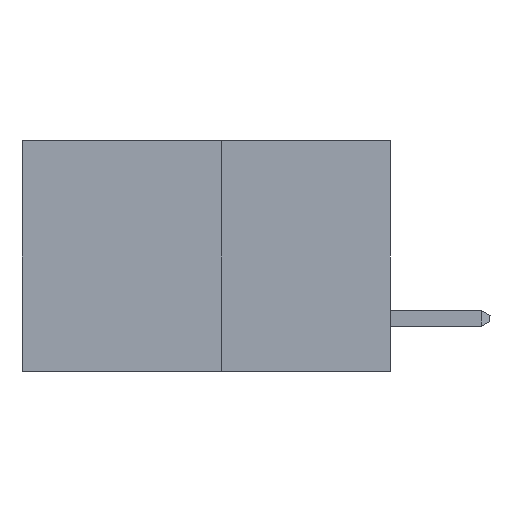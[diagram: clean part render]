
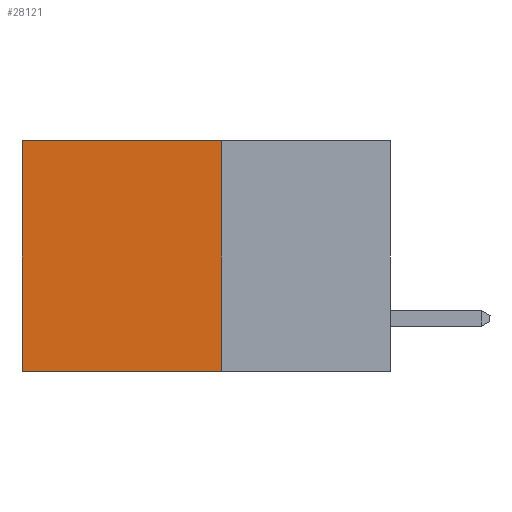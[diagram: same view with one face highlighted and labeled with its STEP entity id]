
A CAD part, left-side view. The second image highlights one B-rep face of the part: STEP entity #28121.
In plain terms, the highlighted planar face has unit normal (-1, 0, 0).
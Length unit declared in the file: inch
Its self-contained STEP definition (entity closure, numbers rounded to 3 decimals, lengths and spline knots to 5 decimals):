
#1997 = LINE ( 'NONE', #16569, #19466 ) ;
#2422 = DIRECTION ( 'NONE',  ( 0., 0., -1. ) ) ;
#3485 = CARTESIAN_POINT ( 'NONE',  ( 0.277, 0.59, 0. ) ) ;
#4413 = VERTEX_POINT ( 'NONE', #3485 ) ;
#4706 = CARTESIAN_POINT ( 'NONE',  ( 0.277, 0.27, -0.37 ) ) ;
#4904 = ORIENTED_EDGE ( 'NONE', *, *, #22801, .F. ) ;
#6611 = VERTEX_POINT ( 'NONE', #9168 ) ;
#7695 = CARTESIAN_POINT ( 'NONE',  ( 0.277, 0.27, -0.37 ) ) ;
#7754 = VERTEX_POINT ( 'NONE', #12438 ) ;
#8692 = EDGE_LOOP ( 'NONE', ( #22581, #11255, #4904, #27289 ) ) ;
#9168 = CARTESIAN_POINT ( 'NONE',  ( 0.277, 0.59, -0.37 ) ) ;
#9518 = CARTESIAN_POINT ( 'NONE',  ( 0.277, 0.59, -0.37 ) ) ;
#10011 = DIRECTION ( 'NONE',  ( 0., 1., 0. ) ) ;
#10153 = LINE ( 'NONE', #9518, #21510 ) ;
#11255 = ORIENTED_EDGE ( 'NONE', *, *, #15597, .F. ) ;
#12438 = CARTESIAN_POINT ( 'NONE',  ( 0.277, 0.27, -0.37 ) ) ;
#13337 = LINE ( 'NONE', #7695, #24687 ) ;
#14248 = DIRECTION ( 'NONE',  ( 0., 0., -1. ) ) ;
#14256 = CARTESIAN_POINT ( 'NONE',  ( 0.277, 0.27, 0. ) ) ;
#15376 = AXIS2_PLACEMENT_3D ( 'NONE', #18698, #27862, #14248 ) ;
#15597 = EDGE_CURVE ( 'NONE', #7754, #6611, #13337, .T. ) ;
#16569 = CARTESIAN_POINT ( 'NONE',  ( 0.277, 0.27, 0. ) ) ;
#17642 = VERTEX_POINT ( 'NONE', #14256 ) ;
#18698 = CARTESIAN_POINT ( 'NONE',  ( 0.277, 0.27, -0.37 ) ) ;
#18823 = DIRECTION ( 'NONE',  ( 0., 1., 0. ) ) ;
#19466 = VECTOR ( 'NONE', #18823, 39.37008 ) ;
#20769 = LINE ( 'NONE', #4706, #26132 ) ;
#20772 = EDGE_CURVE ( 'NONE', #17642, #4413, #1997, .T. ) ;
#21510 = VECTOR ( 'NONE', #25422, 39.37008 ) ;
#21965 = EDGE_CURVE ( 'NONE', #4413, #6611, #10153, .T. ) ;
#22581 = ORIENTED_EDGE ( 'NONE', *, *, #21965, .T. ) ;
#22801 = EDGE_CURVE ( 'NONE', #17642, #7754, #20769, .T. ) ;
#24246 = FACE_OUTER_BOUND ( 'NONE', #8692, .T. ) ;
#24687 = VECTOR ( 'NONE', #10011, 39.37008 ) ;
#25422 = DIRECTION ( 'NONE',  ( 0., 0., -1. ) ) ;
#25557 = PLANE ( 'NONE',  #15376 ) ;
#26132 = VECTOR ( 'NONE', #2422, 39.37008 ) ;
#27289 = ORIENTED_EDGE ( 'NONE', *, *, #20772, .T. ) ;
#27862 = DIRECTION ( 'NONE',  ( 1., 0., 0. ) ) ;
#28121 = ADVANCED_FACE ( 'NONE', ( #24246 ), #25557, .F. ) ;
